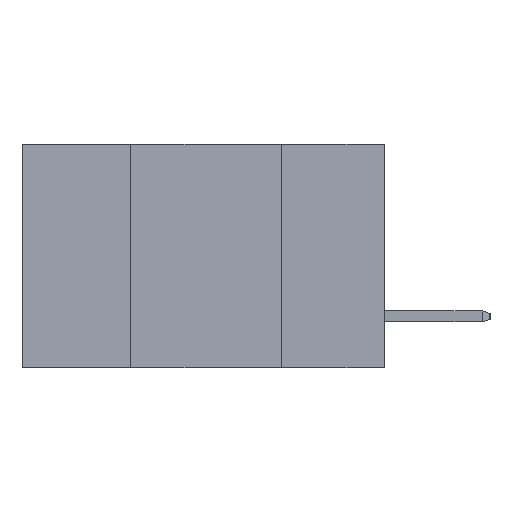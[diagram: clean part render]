
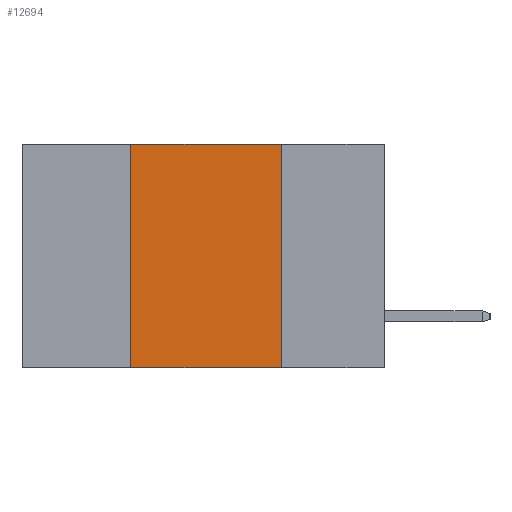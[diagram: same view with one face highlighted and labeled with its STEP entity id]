
A CAD part, left-side view. The second image highlights one B-rep face of the part: STEP entity #12694.
In plain terms, the highlighted planar face has unit normal (-1, 0, 0).
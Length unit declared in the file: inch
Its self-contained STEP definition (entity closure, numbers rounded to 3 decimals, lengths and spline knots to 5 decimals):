
#68 = ORIENTED_EDGE ( 'NONE', *, *, #18391, .T. ) ;
#101 = DIRECTION ( 'NONE',  ( 0., -1., 0. ) ) ;
#114 = CARTESIAN_POINT ( 'NONE',  ( 0., 0.42, -0.37 ) ) ;
#467 = CARTESIAN_POINT ( 'NONE',  ( 0., 0.42, 0. ) ) ;
#1107 = VECTOR ( 'NONE', #2974, 39.37008 ) ;
#1551 = EDGE_LOOP ( 'NONE', ( #3273, #2263, #17569, #68 ) ) ;
#1623 = VERTEX_POINT ( 'NONE', #5097 ) ;
#1725 = LINE ( 'NONE', #18920, #9899 ) ;
#2236 = LINE ( 'NONE', #11504, #14802 ) ;
#2263 = ORIENTED_EDGE ( 'NONE', *, *, #11738, .F. ) ;
#2272 = PLANE ( 'NONE',  #9298 ) ;
#2974 = DIRECTION ( 'NONE',  ( 0., 0., 1. ) ) ;
#3113 = EDGE_CURVE ( 'NONE', #4537, #4974, #5490, .T. ) ;
#3273 = ORIENTED_EDGE ( 'NONE', *, *, #6709, .F. ) ;
#3349 = CARTESIAN_POINT ( 'NONE',  ( 0., 0.42, -0.37 ) ) ;
#4537 = VERTEX_POINT ( 'NONE', #114 ) ;
#4974 = VERTEX_POINT ( 'NONE', #467 ) ;
#5097 = CARTESIAN_POINT ( 'NONE',  ( 0., 0.17, -0.37 ) ) ;
#5490 = LINE ( 'NONE', #3349, #1107 ) ;
#5561 = DIRECTION ( 'NONE',  ( 1., 0., 0. ) ) ;
#6273 = FACE_OUTER_BOUND ( 'NONE', #1551, .T. ) ;
#6709 = EDGE_CURVE ( 'NONE', #21102, #1623, #1725, .T. ) ;
#8096 = CARTESIAN_POINT ( 'NONE',  ( 0., 0.6, 0. ) ) ;
#9298 = AXIS2_PLACEMENT_3D ( 'NONE', #15377, #5561, #17065 ) ;
#9899 = VECTOR ( 'NONE', #18716, 39.37008 ) ;
#11504 = CARTESIAN_POINT ( 'NONE',  ( 0., 0.6, -0.37 ) ) ;
#11738 = EDGE_CURVE ( 'NONE', #4974, #21102, #13248, .T. ) ;
#12694 = ADVANCED_FACE ( 'NONE', ( #6273 ), #2272, .F. ) ;
#13026 = DIRECTION ( 'NONE',  ( 0., -1., 0. ) ) ;
#13248 = LINE ( 'NONE', #8096, #16110 ) ;
#14802 = VECTOR ( 'NONE', #101, 39.37008 ) ;
#15377 = CARTESIAN_POINT ( 'NONE',  ( 0., 0.6, 0. ) ) ;
#16110 = VECTOR ( 'NONE', #13026, 39.37008 ) ;
#16513 = CARTESIAN_POINT ( 'NONE',  ( 0., 0.17, 0. ) ) ;
#17065 = DIRECTION ( 'NONE',  ( 0., 0., -1. ) ) ;
#17569 = ORIENTED_EDGE ( 'NONE', *, *, #3113, .F. ) ;
#18391 = EDGE_CURVE ( 'NONE', #4537, #1623, #2236, .T. ) ;
#18716 = DIRECTION ( 'NONE',  ( 0., 0., -1. ) ) ;
#18920 = CARTESIAN_POINT ( 'NONE',  ( 0., 0.17, -0.37 ) ) ;
#21102 = VERTEX_POINT ( 'NONE', #16513 ) ;
